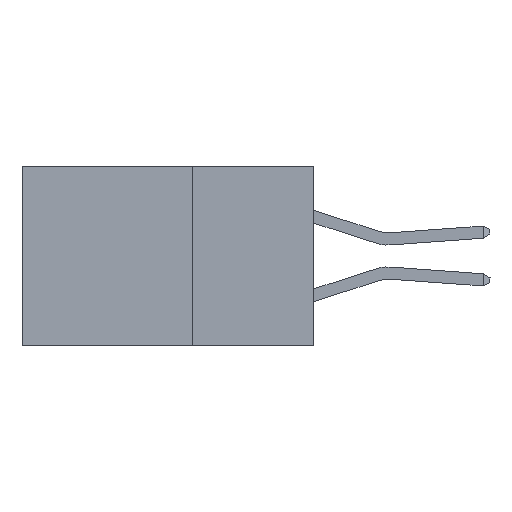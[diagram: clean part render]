
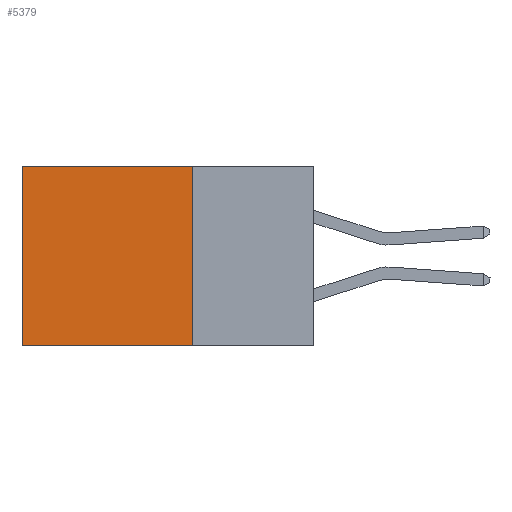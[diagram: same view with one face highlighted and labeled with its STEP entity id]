
A CAD part, left-side view. The second image highlights one B-rep face of the part: STEP entity #5379.
In plain terms, the highlighted planar face has unit normal (-1, 0, 0).
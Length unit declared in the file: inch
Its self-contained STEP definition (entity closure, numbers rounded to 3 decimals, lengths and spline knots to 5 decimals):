
#277 = CARTESIAN_POINT ( 'NONE',  ( 0.2875, 0.25, 0. ) ) ;
#1515 = CARTESIAN_POINT ( 'NONE',  ( 0.2875, 0.6, 0. ) ) ;
#3215 = EDGE_CURVE ( 'NONE', #34707, #18679, #18124, .T. ) ;
#3270 = EDGE_CURVE ( 'NONE', #8212, #18679, #6464, .T. ) ;
#4823 = CARTESIAN_POINT ( 'NONE',  ( 0.2875, 0.25, 0. ) ) ;
#5379 = ADVANCED_FACE ( 'NONE', ( #20101 ), #24317, .F. ) ;
#6026 = VECTOR ( 'NONE', #9747, 39.37008 ) ;
#6391 = EDGE_CURVE ( 'NONE', #26064, #34707, #13594, .T. ) ;
#6464 = LINE ( 'NONE', #31853, #6026 ) ;
#6733 = ORIENTED_EDGE ( 'NONE', *, *, #11893, .F. ) ;
#7598 = VECTOR ( 'NONE', #15895, 39.37008 ) ;
#8212 = VERTEX_POINT ( 'NONE', #35049 ) ;
#8338 = LINE ( 'NONE', #32271, #25117 ) ;
#9747 = DIRECTION ( 'NONE',  ( 0., 1., 0. ) ) ;
#11893 = EDGE_CURVE ( 'NONE', #26064, #8212, #8338, .T. ) ;
#12026 = VECTOR ( 'NONE', #15249, 39.37008 ) ;
#13323 = DIRECTION ( 'NONE',  ( 1., 0., 0. ) ) ;
#13594 = LINE ( 'NONE', #4823, #7598 ) ;
#15249 = DIRECTION ( 'NONE',  ( 0., 0., -1. ) ) ;
#15895 = DIRECTION ( 'NONE',  ( 0., 1., 0. ) ) ;
#18124 = LINE ( 'NONE', #23495, #12026 ) ;
#18679 = VERTEX_POINT ( 'NONE', #24436 ) ;
#19251 = ORIENTED_EDGE ( 'NONE', *, *, #3215, .T. ) ;
#19911 = ORIENTED_EDGE ( 'NONE', *, *, #3270, .F. ) ;
#20101 = FACE_OUTER_BOUND ( 'NONE', #28314, .T. ) ;
#21355 = DIRECTION ( 'NONE',  ( 0., 0., -1. ) ) ;
#21429 = CARTESIAN_POINT ( 'NONE',  ( 0.2875, 0.25, 0. ) ) ;
#23495 = CARTESIAN_POINT ( 'NONE',  ( 0.2875, 0.6, 0. ) ) ;
#24317 = PLANE ( 'NONE',  #27527 ) ;
#24436 = CARTESIAN_POINT ( 'NONE',  ( 0.2875, 0.6, -0.37 ) ) ;
#25117 = VECTOR ( 'NONE', #21355, 39.37008 ) ;
#26064 = VERTEX_POINT ( 'NONE', #277 ) ;
#27208 = DIRECTION ( 'NONE',  ( 0., 0., -1. ) ) ;
#27527 = AXIS2_PLACEMENT_3D ( 'NONE', #21429, #13323, #27208 ) ;
#28314 = EDGE_LOOP ( 'NONE', ( #19251, #19911, #6733, #33438 ) ) ;
#31853 = CARTESIAN_POINT ( 'NONE',  ( 0.2875, 0.25, -0.37 ) ) ;
#32271 = CARTESIAN_POINT ( 'NONE',  ( 0.2875, 0.25, 0. ) ) ;
#33438 = ORIENTED_EDGE ( 'NONE', *, *, #6391, .T. ) ;
#34707 = VERTEX_POINT ( 'NONE', #1515 ) ;
#35049 = CARTESIAN_POINT ( 'NONE',  ( 0.2875, 0.25, -0.37 ) ) ;
